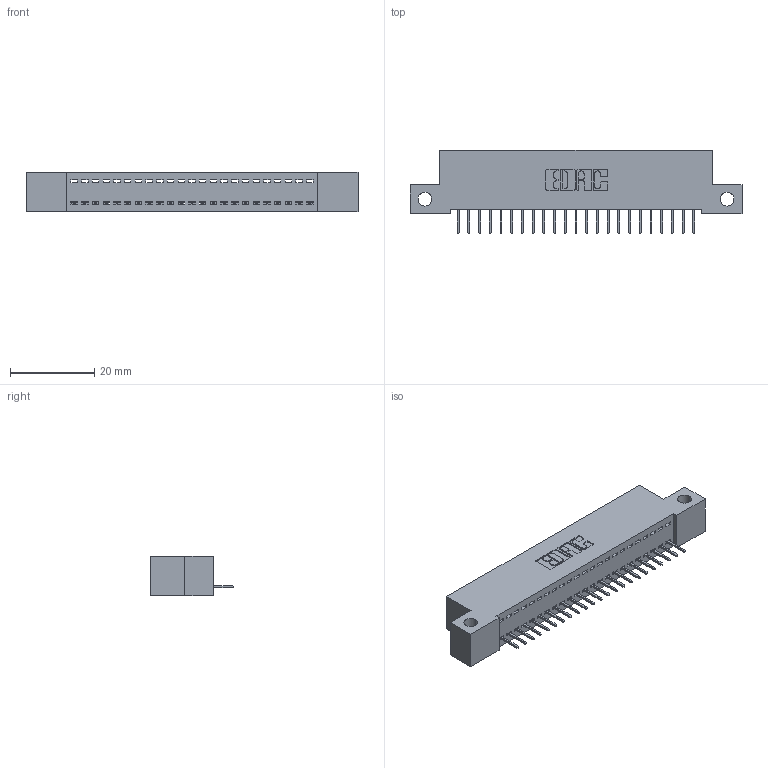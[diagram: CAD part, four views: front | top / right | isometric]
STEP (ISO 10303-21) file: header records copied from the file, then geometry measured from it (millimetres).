
FILE_DESCRIPTION (( 'STEP AP203' ), '1' );
FILE_NAME ('392-023-524-112.STEP', '2018-08-15T13:25:50', ( '' ), ( '' ), 'SwSTEP 2.0', 'SolidWorks 2016', '' );
FILE_SCHEMA (( 'CONFIG_CONTROL_DESIGN' ));
Length unit declared in the file: inch
Products named in the file (3): 342 Part_Side Mount; 345-292-001_345-293-124; 392-023-524-112
Assembly tree (24 placements, depth 2):
  392-023-524-112
    342 Part_Side Mount
    345-292-001_345-293-124  x23
Bounding box: 78.74 x 19.69 x 9.4 mm (x, y, z)
Volume: 6669.2 mm3; surface area: 8993.3 mm2
Topology: 24 solids, 24 shells, 1536 faces, 4439 edges, 2866 vertices
Faces by surface type: plane 1170, cylinder 366
Entity records: 16463 total; most frequent: CARTESIAN_POINT 2847, ORIENTED_EDGE 2806, DIRECTION 2441, EDGE_CURVE 1403, VECTOR 1279, LINE 1279, VERTEX_POINT 930, AXIS2_PLACEMENT_3D 581
